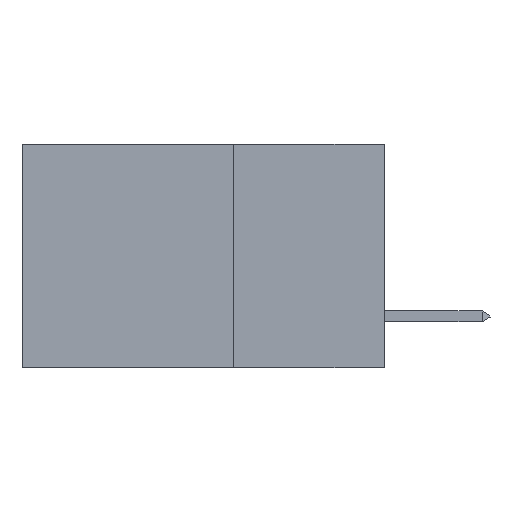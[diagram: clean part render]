
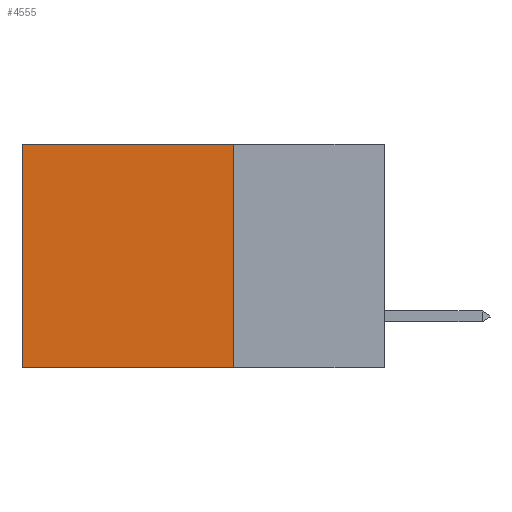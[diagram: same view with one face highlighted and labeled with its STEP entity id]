
A CAD part, left-side view. The second image highlights one B-rep face of the part: STEP entity #4555.
In plain terms, the highlighted planar face has unit normal (-1, 0, 0).
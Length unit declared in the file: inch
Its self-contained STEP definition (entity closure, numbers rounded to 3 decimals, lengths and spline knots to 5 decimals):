
#93 = CARTESIAN_POINT ( 'NONE',  ( 0.2875, 0.6, 0. ) ) ;
#336 = EDGE_LOOP ( 'NONE', ( #1318, #5792, #2713, #888 ) ) ;
#454 = VECTOR ( 'NONE', #1034, 39.37008 ) ;
#666 = DIRECTION ( 'NONE',  ( 0., 0., -1. ) ) ;
#722 = CARTESIAN_POINT ( 'NONE',  ( 0.2875, 0.25, -0.37 ) ) ;
#888 = ORIENTED_EDGE ( 'NONE', *, *, #5755, .T. ) ;
#988 = VERTEX_POINT ( 'NONE', #2810 ) ;
#1034 = DIRECTION ( 'NONE',  ( 0., 1., 0. ) ) ;
#1318 = ORIENTED_EDGE ( 'NONE', *, *, #5453, .T. ) ;
#1589 = EDGE_CURVE ( 'NONE', #988, #2409, #8643, .T. ) ;
#1704 = VECTOR ( 'NONE', #7188, 39.37008 ) ;
#1909 = CARTESIAN_POINT ( 'NONE',  ( 0.2875, 0.6, -0.37 ) ) ;
#2089 = PLANE ( 'NONE',  #2521 ) ;
#2409 = VERTEX_POINT ( 'NONE', #722 ) ;
#2521 = AXIS2_PLACEMENT_3D ( 'NONE', #4052, #2904, #2809 ) ;
#2656 = VECTOR ( 'NONE', #7469, 39.37008 ) ;
#2713 = ORIENTED_EDGE ( 'NONE', *, *, #1589, .F. ) ;
#2809 = DIRECTION ( 'NONE',  ( 0., 0., -1. ) ) ;
#2810 = CARTESIAN_POINT ( 'NONE',  ( 0.2875, 0.25, 0. ) ) ;
#2904 = DIRECTION ( 'NONE',  ( 1., 0., 0. ) ) ;
#3124 = CARTESIAN_POINT ( 'NONE',  ( 0.2875, 0.6, 0. ) ) ;
#3226 = VERTEX_POINT ( 'NONE', #1909 ) ;
#3346 = CARTESIAN_POINT ( 'NONE',  ( 0.2875, 0.25, 0. ) ) ;
#3495 = LINE ( 'NONE', #3124, #1704 ) ;
#4052 = CARTESIAN_POINT ( 'NONE',  ( 0.2875, 0.25, 0. ) ) ;
#4205 = EDGE_CURVE ( 'NONE', #2409, #3226, #8468, .T. ) ;
#4517 = CARTESIAN_POINT ( 'NONE',  ( 0.2875, 0.25, -0.37 ) ) ;
#4555 = ADVANCED_FACE ( 'NONE', ( #5351 ), #2089, .F. ) ;
#4784 = CARTESIAN_POINT ( 'NONE',  ( 0.2875, 0.25, 0. ) ) ;
#4999 = LINE ( 'NONE', #4784, #2656 ) ;
#5351 = FACE_OUTER_BOUND ( 'NONE', #336, .T. ) ;
#5453 = EDGE_CURVE ( 'NONE', #7950, #3226, #3495, .T. ) ;
#5755 = EDGE_CURVE ( 'NONE', #988, #7950, #4999, .T. ) ;
#5792 = ORIENTED_EDGE ( 'NONE', *, *, #4205, .F. ) ;
#7188 = DIRECTION ( 'NONE',  ( 0., 0., -1. ) ) ;
#7469 = DIRECTION ( 'NONE',  ( 0., 1., 0. ) ) ;
#7675 = VECTOR ( 'NONE', #666, 39.37008 ) ;
#7950 = VERTEX_POINT ( 'NONE', #93 ) ;
#8468 = LINE ( 'NONE', #4517, #454 ) ;
#8643 = LINE ( 'NONE', #3346, #7675 ) ;
